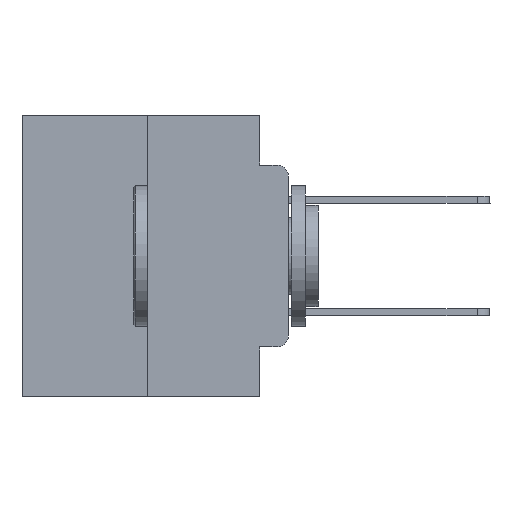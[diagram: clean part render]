
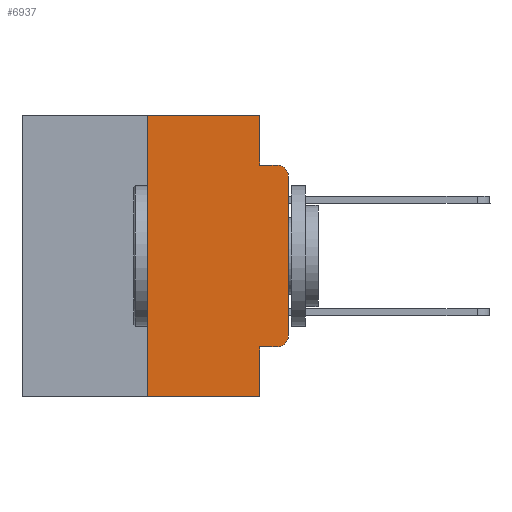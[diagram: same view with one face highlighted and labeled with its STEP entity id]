
A CAD part, left-side view. The second image highlights one B-rep face of the part: STEP entity #6937.
In plain terms, the highlighted planar face has unit normal (-1, 0, 0).
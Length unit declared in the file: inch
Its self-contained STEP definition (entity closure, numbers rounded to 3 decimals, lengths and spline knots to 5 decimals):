
#196 = EDGE_CURVE ( 'NONE', #7732, #26016, #18031, .T. ) ;
#889 = EDGE_CURVE ( 'NONE', #21102, #21805, #8952, .T. ) ;
#929 = EDGE_CURVE ( 'NONE', #6591, #23586, #23992, .T. ) ;
#2066 = DIRECTION ( 'NONE',  ( 0., -1., 0. ) ) ;
#2623 = DIRECTION ( 'NONE',  ( 0., 0., -1. ) ) ;
#2641 = CARTESIAN_POINT ( 'NONE',  ( 0., 0.25, -0.5 ) ) ;
#3064 = DIRECTION ( 'NONE',  ( 0., 0., 1. ) ) ;
#3123 = CARTESIAN_POINT ( 'NONE',  ( 0., 0.051, -0.4115 ) ) ;
#3485 = VERTEX_POINT ( 'NONE', #12274 ) ;
#3487 = AXIS2_PLACEMENT_3D ( 'NONE', #21538, #6592, #13041 ) ;
#3649 = VERTEX_POINT ( 'NONE', #17111 ) ;
#3973 = VECTOR ( 'NONE', #5166, 39.37008 ) ;
#4435 = PLANE ( 'NONE',  #3487 ) ;
#4769 = ORIENTED_EDGE ( 'NONE', *, *, #18465, .T. ) ;
#4857 = CARTESIAN_POINT ( 'NONE',  ( 0., 0.051, 0. ) ) ;
#5166 = DIRECTION ( 'NONE',  ( 0., -1., 0. ) ) ;
#5262 = EDGE_CURVE ( 'NONE', #24015, #7732, #11074, .T. ) ;
#5481 = EDGE_CURVE ( 'NONE', #23586, #3485, #15387, .T. ) ;
#5822 = DIRECTION ( 'NONE',  ( 0., 0., -1. ) ) ;
#6250 = DIRECTION ( 'NONE',  ( 0., 0., 1. ) ) ;
#6328 = ORIENTED_EDGE ( 'NONE', *, *, #929, .T. ) ;
#6591 = VERTEX_POINT ( 'NONE', #9887 ) ;
#6592 = DIRECTION ( 'NONE',  ( 1., 0., 0. ) ) ;
#6633 = ORIENTED_EDGE ( 'NONE', *, *, #21080, .T. ) ;
#6695 = VECTOR ( 'NONE', #2623, 39.37008 ) ;
#6937 = ADVANCED_FACE ( 'NONE', ( #23745 ), #4435, .F. ) ;
#7732 = VERTEX_POINT ( 'NONE', #21845 ) ;
#8952 = LINE ( 'NONE', #25127, #23647 ) ;
#9727 = VECTOR ( 'NONE', #6250, 39.37008 ) ;
#9887 = CARTESIAN_POINT ( 'NONE',  ( 0., 0.02, -0.4115 ) ) ;
#9921 = DIRECTION ( 'NONE',  ( 0., -1., 0. ) ) ;
#9945 = VERTEX_POINT ( 'NONE', #16805 ) ;
#10610 = AXIS2_PLACEMENT_3D ( 'NONE', #19592, #15475, #15380 ) ;
#11074 = LINE ( 'NONE', #19062, #9727 ) ;
#11178 = CARTESIAN_POINT ( 'NONE',  ( 0., 0.051, -0.0885 ) ) ;
#12045 = EDGE_CURVE ( 'NONE', #3649, #6591, #26492, .T. ) ;
#12053 = VECTOR ( 'NONE', #3064, 39.37008 ) ;
#12274 = CARTESIAN_POINT ( 'NONE',  ( 0., 0., -0.1085 ) ) ;
#12598 = EDGE_CURVE ( 'NONE', #3649, #9945, #23740, .T. ) ;
#12721 = CARTESIAN_POINT ( 'NONE',  ( 0., 0.473, -0.5 ) ) ;
#12769 = CIRCLE ( 'NONE', #10610, 0.02 ) ;
#13041 = DIRECTION ( 'NONE',  ( 0., 0., -1. ) ) ;
#13215 = VECTOR ( 'NONE', #21370, 39.37008 ) ;
#13587 = ORIENTED_EDGE ( 'NONE', *, *, #5481, .T. ) ;
#13701 = CARTESIAN_POINT ( 'NONE',  ( 0., 0., -0.3915 ) ) ;
#14411 = VECTOR ( 'NONE', #2066, 39.37008 ) ;
#15176 = AXIS2_PLACEMENT_3D ( 'NONE', #20588, #22723, #5822 ) ;
#15380 = DIRECTION ( 'NONE',  ( 0., 0., -1. ) ) ;
#15387 = LINE ( 'NONE', #19987, #12053 ) ;
#15475 = DIRECTION ( 'NONE',  ( -1., 0., 0. ) ) ;
#15566 = DIRECTION ( 'NONE',  ( 0., -1., 0. ) ) ;
#16805 = CARTESIAN_POINT ( 'NONE',  ( 0., 0.051, -0.5 ) ) ;
#17111 = CARTESIAN_POINT ( 'NONE',  ( 0., 0.051, -0.4115 ) ) ;
#17351 = EDGE_LOOP ( 'NONE', ( #13587, #6633, #21332, #24895, #21357, #26276, #4769, #18466, #23528, #6328 ) ) ;
#17675 = CARTESIAN_POINT ( 'NONE',  ( 0., 0.02, -0.0885 ) ) ;
#17793 = CARTESIAN_POINT ( 'NONE',  ( 0., 0.051, 0. ) ) ;
#18031 = LINE ( 'NONE', #18075, #3973 ) ;
#18075 = CARTESIAN_POINT ( 'NONE',  ( 0., 0.473, 0. ) ) ;
#18465 = EDGE_CURVE ( 'NONE', #24015, #9945, #24758, .T. ) ;
#18466 = ORIENTED_EDGE ( 'NONE', *, *, #12598, .F. ) ;
#19062 = CARTESIAN_POINT ( 'NONE',  ( 0., 0.25, 0. ) ) ;
#19117 = EDGE_CURVE ( 'NONE', #26016, #21102, #23248, .T. ) ;
#19492 = VECTOR ( 'NONE', #15566, 39.37008 ) ;
#19592 = CARTESIAN_POINT ( 'NONE',  ( 0., 0.02, -0.1085 ) ) ;
#19987 = CARTESIAN_POINT ( 'NONE',  ( 0., 0., 0. ) ) ;
#20588 = CARTESIAN_POINT ( 'NONE',  ( 0., 0.02, -0.3915 ) ) ;
#21080 = EDGE_CURVE ( 'NONE', #3485, #21805, #12769, .T. ) ;
#21102 = VERTEX_POINT ( 'NONE', #11178 ) ;
#21332 = ORIENTED_EDGE ( 'NONE', *, *, #889, .F. ) ;
#21357 = ORIENTED_EDGE ( 'NONE', *, *, #196, .F. ) ;
#21370 = DIRECTION ( 'NONE',  ( 0., 0., -1. ) ) ;
#21538 = CARTESIAN_POINT ( 'NONE',  ( 0., 0.473, 0. ) ) ;
#21805 = VERTEX_POINT ( 'NONE', #17675 ) ;
#21845 = CARTESIAN_POINT ( 'NONE',  ( 0., 0.25, 0. ) ) ;
#22723 = DIRECTION ( 'NONE',  ( -1., 0., 0. ) ) ;
#23248 = LINE ( 'NONE', #25657, #13215 ) ;
#23528 = ORIENTED_EDGE ( 'NONE', *, *, #12045, .T. ) ;
#23586 = VERTEX_POINT ( 'NONE', #13701 ) ;
#23647 = VECTOR ( 'NONE', #9921, 39.37008 ) ;
#23740 = LINE ( 'NONE', #4857, #6695 ) ;
#23745 = FACE_OUTER_BOUND ( 'NONE', #17351, .T. ) ;
#23992 = CIRCLE ( 'NONE', #15176, 0.02 ) ;
#24015 = VERTEX_POINT ( 'NONE', #2641 ) ;
#24758 = LINE ( 'NONE', #12721, #14411 ) ;
#24895 = ORIENTED_EDGE ( 'NONE', *, *, #19117, .F. ) ;
#25127 = CARTESIAN_POINT ( 'NONE',  ( 0., 0.051, -0.0885 ) ) ;
#25657 = CARTESIAN_POINT ( 'NONE',  ( 0., 0.051, 0. ) ) ;
#26016 = VERTEX_POINT ( 'NONE', #17793 ) ;
#26276 = ORIENTED_EDGE ( 'NONE', *, *, #5262, .F. ) ;
#26492 = LINE ( 'NONE', #3123, #19492 ) ;
